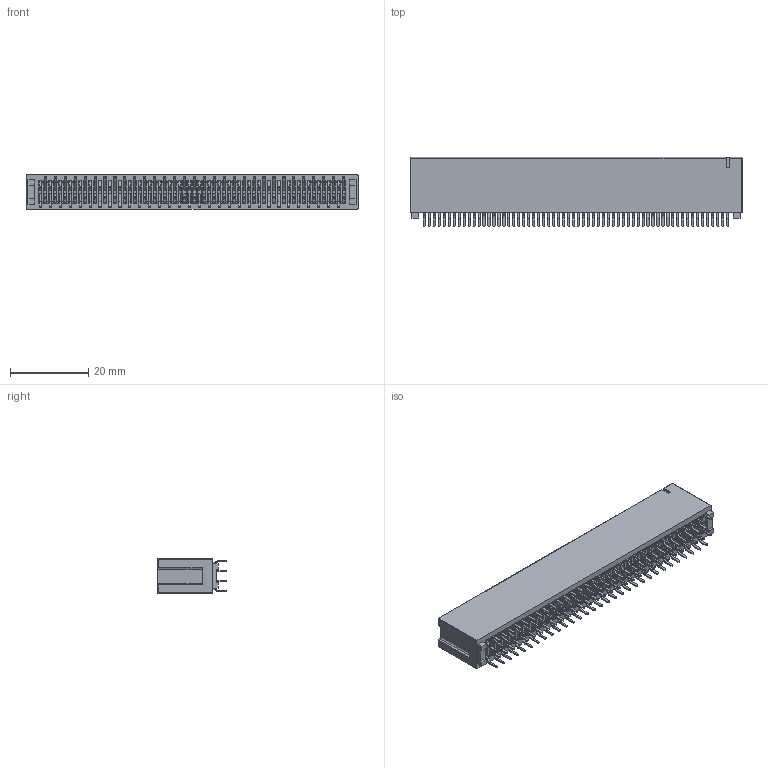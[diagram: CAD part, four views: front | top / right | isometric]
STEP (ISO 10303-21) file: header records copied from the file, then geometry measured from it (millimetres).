
FILE_DESCRIPTION (( 'STEP AP203' ), '1' );
FILE_NAME ('302-124-621-201.STEP', '2024-04-01T19:39:37', ( '' ), ( '' ), 'SwSTEP 2.0', 'SolidWorks 2023', '' );
FILE_SCHEMA (( 'CONFIG_CONTROL_DESIGN' ));
Length unit declared in the file: millimetre
Products named in the file (4): Contact_302-290-X21 (2); Contact_302-290-X21 (1); 302-124-621-201; HSG_Vertical HSG
Assembly tree (125 placements, depth 2):
  302-124-621-201
    HSG_Vertical HSG
    Contact_302-290-X21 (2)  x62
    Contact_302-290-X21 (1)  x62
Bounding box: 84.84 x 17.63 x 8.88 mm (x, y, z)
Volume: 6440.1 mm3; surface area: 18527.2 mm2
Topology: 125 solids, 125 shells, 5708 faces, 16784 edges, 11016 vertices
Faces by surface type: plane 4203, cylinder 1253, bspline 248, sphere 4
Entity records: 47516 total; most frequent: ORIENTED_EDGE 8184, CARTESIAN_POINT 8116, DIRECTION 6542, EDGE_CURVE 4092, VECTOR 4018, LINE 4018, VERTEX_POINT 2720, AXIS2_PLACEMENT_3D 1262
